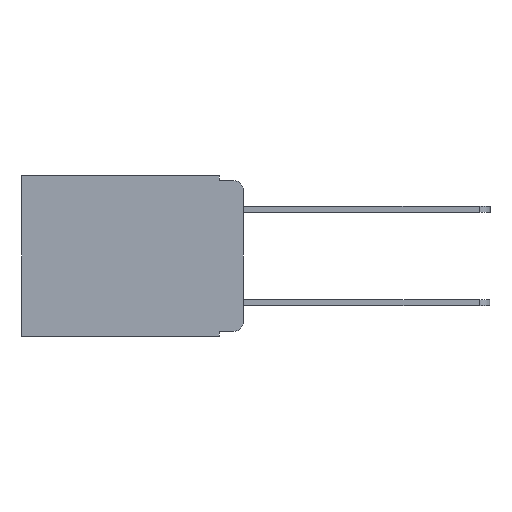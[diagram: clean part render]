
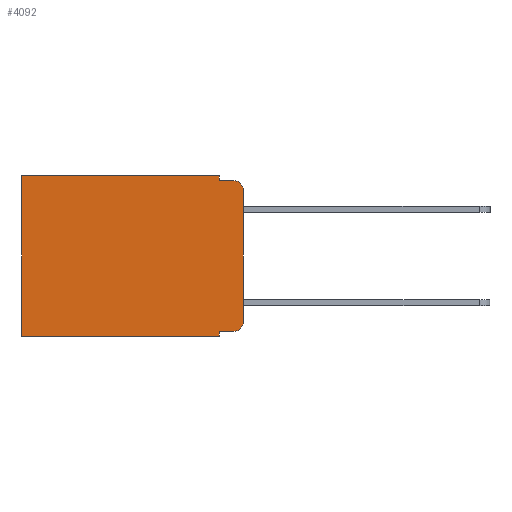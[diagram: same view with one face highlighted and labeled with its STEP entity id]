
A CAD part, left-side view. The second image highlights one B-rep face of the part: STEP entity #4092.
In plain terms, the highlighted planar face has unit normal (-1, 0, 0).
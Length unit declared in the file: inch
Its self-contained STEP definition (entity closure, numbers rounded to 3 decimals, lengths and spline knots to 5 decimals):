
#37 = VERTEX_POINT ( 'NONE', #7791 ) ;
#40 = AXIS2_PLACEMENT_3D ( 'NONE', #367, #6188, #5684 ) ;
#68 = EDGE_CURVE ( 'NONE', #5789, #7959, #1240, .T. ) ;
#79 = LINE ( 'NONE', #9435, #8661 ) ;
#112 = EDGE_CURVE ( 'NONE', #37, #6919, #975, .T. ) ;
#164 = ORIENTED_EDGE ( 'NONE', *, *, #9084, .T. ) ;
#299 = LINE ( 'NONE', #1878, #4511 ) ;
#310 = CARTESIAN_POINT ( 'NONE',  ( 0.298, 0.051, -0.01 ) ) ;
#367 = CARTESIAN_POINT ( 'NONE',  ( 0.298, 0.02, -0.313 ) ) ;
#491 = VERTEX_POINT ( 'NONE', #310 ) ;
#522 = ORIENTED_EDGE ( 'NONE', *, *, #1020, .F. ) ;
#567 = EDGE_CURVE ( 'NONE', #844, #5770, #2700, .T. ) ;
#680 = CARTESIAN_POINT ( 'NONE',  ( 0.298, 0., -0.313 ) ) ;
#685 = CARTESIAN_POINT ( 'NONE',  ( 0.298, 0.02, -0.333 ) ) ;
#837 = EDGE_CURVE ( 'NONE', #1274, #6414, #6914, .T. ) ;
#844 = VERTEX_POINT ( 'NONE', #1631 ) ;
#975 = LINE ( 'NONE', #7552, #3224 ) ;
#1020 = EDGE_CURVE ( 'NONE', #491, #5770, #7584, .T. ) ;
#1240 = LINE ( 'NONE', #3773, #3473 ) ;
#1274 = VERTEX_POINT ( 'NONE', #685 ) ;
#1400 = AXIS2_PLACEMENT_3D ( 'NONE', #6932, #7157, #7623 ) ;
#1552 = CARTESIAN_POINT ( 'NONE',  ( 0.298, 0.051, -0.01 ) ) ;
#1631 = CARTESIAN_POINT ( 'NONE',  ( 0.298, 0., -0.03 ) ) ;
#1878 = CARTESIAN_POINT ( 'NONE',  ( 0.298, 0.051, 0. ) ) ;
#2224 = DIRECTION ( 'NONE',  ( 0., -1., 0. ) ) ;
#2281 = EDGE_CURVE ( 'NONE', #5776, #1274, #3736, .T. ) ;
#2446 = EDGE_CURVE ( 'NONE', #5789, #491, #299, .T. ) ;
#2603 = DIRECTION ( 'NONE',  ( 0., 1., 0. ) ) ;
#2700 = CIRCLE ( 'NONE', #1400, 0.02 ) ;
#2755 = ORIENTED_EDGE ( 'NONE', *, *, #837, .T. ) ;
#2761 = CARTESIAN_POINT ( 'NONE',  ( 0.298, 0., 0. ) ) ;
#2933 = CARTESIAN_POINT ( 'NONE',  ( 0.298, 0.051, -0.333 ) ) ;
#2966 = DIRECTION ( 'NONE',  ( 0., 0., -1. ) ) ;
#2980 = DIRECTION ( 'NONE',  ( 1., 0., 0. ) ) ;
#3141 = DIRECTION ( 'NONE',  ( 0., 0., -1. ) ) ;
#3224 = VECTOR ( 'NONE', #2603, 39.37008 ) ;
#3270 = CARTESIAN_POINT ( 'NONE',  ( 0.298, 0.051, 0. ) ) ;
#3473 = VECTOR ( 'NONE', #8694, 39.37008 ) ;
#3484 = VECTOR ( 'NONE', #7415, 39.37008 ) ;
#3736 = LINE ( 'NONE', #3857, #3484 ) ;
#3773 = CARTESIAN_POINT ( 'NONE',  ( 0.298, 0., 0. ) ) ;
#3857 = CARTESIAN_POINT ( 'NONE',  ( 0.298, 0.051, -0.333 ) ) ;
#3975 = ORIENTED_EDGE ( 'NONE', *, *, #112, .F. ) ;
#4092 = ADVANCED_FACE ( 'NONE', ( #10465 ), #6460, .F. ) ;
#4182 = CARTESIAN_POINT ( 'NONE',  ( 0.298, 0.473, 0. ) ) ;
#4360 = CARTESIAN_POINT ( 'NONE',  ( 0.298, 0.473, 0. ) ) ;
#4375 = EDGE_CURVE ( 'NONE', #844, #6414, #7808, .T. ) ;
#4511 = VECTOR ( 'NONE', #5526, 39.37008 ) ;
#5151 = CARTESIAN_POINT ( 'NONE',  ( 0.298, 0., 0. ) ) ;
#5286 = ORIENTED_EDGE ( 'NONE', *, *, #68, .T. ) ;
#5347 = ORIENTED_EDGE ( 'NONE', *, *, #6214, .F. ) ;
#5502 = CARTESIAN_POINT ( 'NONE',  ( 0.298, 0.473, -0.343 ) ) ;
#5526 = DIRECTION ( 'NONE',  ( 0., 0., -1. ) ) ;
#5588 = VECTOR ( 'NONE', #9800, 39.37008 ) ;
#5684 = DIRECTION ( 'NONE',  ( 0., 0., -1. ) ) ;
#5770 = VERTEX_POINT ( 'NONE', #6995 ) ;
#5776 = VERTEX_POINT ( 'NONE', #2933 ) ;
#5789 = VERTEX_POINT ( 'NONE', #3270 ) ;
#5837 = ORIENTED_EDGE ( 'NONE', *, *, #2281, .T. ) ;
#6188 = DIRECTION ( 'NONE',  ( -1., 0., 0. ) ) ;
#6207 = DIRECTION ( 'NONE',  ( 0., 0., -1. ) ) ;
#6214 = EDGE_CURVE ( 'NONE', #5776, #37, #79, .T. ) ;
#6414 = VERTEX_POINT ( 'NONE', #680 ) ;
#6460 = PLANE ( 'NONE',  #9855 ) ;
#6826 = EDGE_LOOP ( 'NONE', ( #9224, #9505, #522, #7586, #5286, #164, #3975, #5347, #5837, #2755 ) ) ;
#6914 = CIRCLE ( 'NONE', #40, 0.02 ) ;
#6919 = VERTEX_POINT ( 'NONE', #5502 ) ;
#6932 = CARTESIAN_POINT ( 'NONE',  ( 0.298, 0.02, -0.03 ) ) ;
#6995 = CARTESIAN_POINT ( 'NONE',  ( 0.298, 0.02, -0.01 ) ) ;
#7157 = DIRECTION ( 'NONE',  ( -1., 0., 0. ) ) ;
#7304 = VECTOR ( 'NONE', #2224, 39.37008 ) ;
#7415 = DIRECTION ( 'NONE',  ( 0., -1., 0. ) ) ;
#7552 = CARTESIAN_POINT ( 'NONE',  ( 0.298, 0., -0.343 ) ) ;
#7584 = LINE ( 'NONE', #1552, #7304 ) ;
#7586 = ORIENTED_EDGE ( 'NONE', *, *, #2446, .F. ) ;
#7623 = DIRECTION ( 'NONE',  ( 0., 0., -1. ) ) ;
#7791 = CARTESIAN_POINT ( 'NONE',  ( 0.298, 0.051, -0.343 ) ) ;
#7796 = LINE ( 'NONE', #4182, #5588 ) ;
#7808 = LINE ( 'NONE', #5151, #9875 ) ;
#7959 = VERTEX_POINT ( 'NONE', #4360 ) ;
#8661 = VECTOR ( 'NONE', #6207, 39.37008 ) ;
#8694 = DIRECTION ( 'NONE',  ( 0., 1., 0. ) ) ;
#9084 = EDGE_CURVE ( 'NONE', #7959, #6919, #7796, .T. ) ;
#9224 = ORIENTED_EDGE ( 'NONE', *, *, #4375, .F. ) ;
#9435 = CARTESIAN_POINT ( 'NONE',  ( 0.298, 0.051, 0. ) ) ;
#9505 = ORIENTED_EDGE ( 'NONE', *, *, #567, .T. ) ;
#9800 = DIRECTION ( 'NONE',  ( 0., 0., -1. ) ) ;
#9855 = AXIS2_PLACEMENT_3D ( 'NONE', #2761, #2980, #2966 ) ;
#9875 = VECTOR ( 'NONE', #3141, 39.37008 ) ;
#10465 = FACE_OUTER_BOUND ( 'NONE', #6826, .T. ) ;
